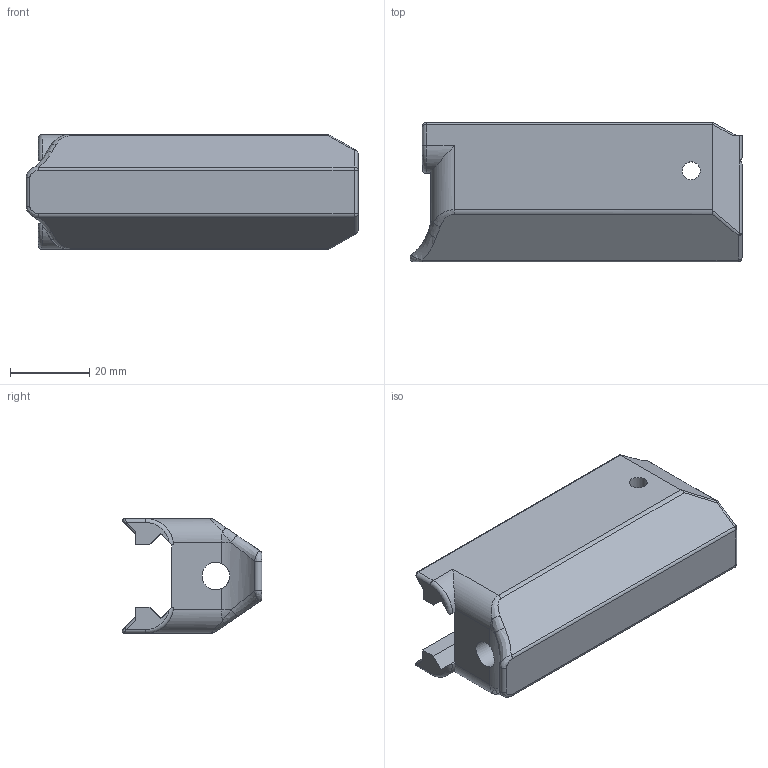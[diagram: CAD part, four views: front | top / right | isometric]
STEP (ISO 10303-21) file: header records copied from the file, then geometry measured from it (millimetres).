
FILE_DESCRIPTION(/* description */ (''),/* implementation_level */ '2;1');
FILE_NAME(/* name */ 'Gros Weight Module.step',/* time_stamp */ '2021-07-12T09:01:25-06:00',/* author */ (''),/* organization */ (''),/* preprocessor_version */ 'ST-DEVELOPER v18.1',/* originating_system */ 'Autodesk Translation Framework v10.9.0.1377',/* authorisation */ '');
FILE_SCHEMA (('AUTOMOTIVE_DESIGN { 1 0 10303 214 3 1 1 }'));
Length unit declared in the file: millimetre
Products named in the file (1): FNS Release
Bounding box: 83.79 x 35.29 x 28.99 mm (x, y, z)
Volume: 46507.8 mm3; surface area: 14977.5 mm2
Topology: 1 solids, 1 shells, 449 faces, 1265 edges, 832 vertices
Faces by surface type: bspline 309, plane 97, cylinder 34, sphere 4, torus 4, cone 1
Full cylindrical faces by diameter (mm): 4.5 x1, 5 x1, 7 x1, 8.6 x1, 9.7 x1
Entity records: 15673 total; most frequent: CARTESIAN_POINT 7013, ORIENTED_EDGE 2530, EDGE_CURVE 1265, DIRECTION 1005, VERTEX_POINT 832, LINE 563, VECTOR 563, EDGE_LOOP 469
